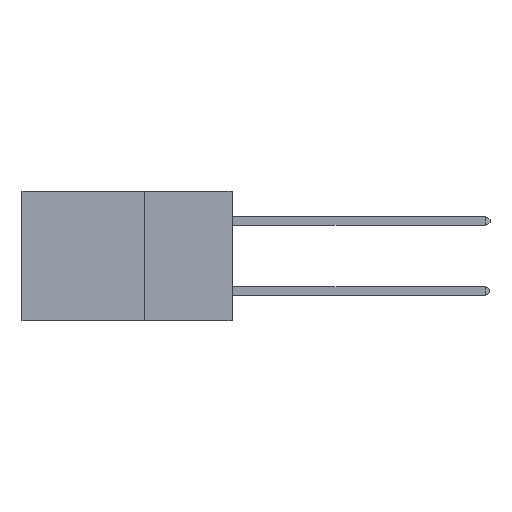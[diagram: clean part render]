
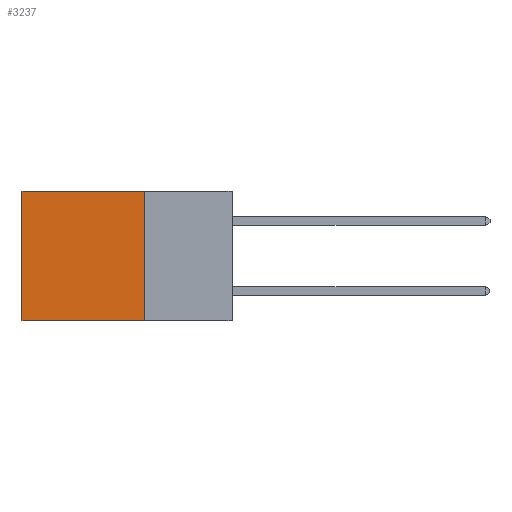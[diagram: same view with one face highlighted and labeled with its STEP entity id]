
A CAD part, left-side view. The second image highlights one B-rep face of the part: STEP entity #3237.
In plain terms, the highlighted planar face has unit normal (-1, 0, 0).
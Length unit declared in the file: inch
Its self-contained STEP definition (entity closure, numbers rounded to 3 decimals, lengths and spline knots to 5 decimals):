
#46 = VERTEX_POINT ( 'NONE', #4002 ) ;
#848 = DIRECTION ( 'NONE',  ( 1., 0., 0. ) ) ;
#983 = VECTOR ( 'NONE', #1542, 39.37008 ) ;
#1263 = VERTEX_POINT ( 'NONE', #14115 ) ;
#1542 = DIRECTION ( 'NONE',  ( 0., 0., -1. ) ) ;
#1640 = EDGE_LOOP ( 'NONE', ( #15507, #9626, #14512, #6989 ) ) ;
#1706 = EDGE_CURVE ( 'NONE', #14090, #1263, #13943, .T. ) ;
#1722 = VECTOR ( 'NONE', #9098, 39.37008 ) ;
#2102 = LINE ( 'NONE', #12699, #1722 ) ;
#3237 = ADVANCED_FACE ( 'NONE', ( #11643 ), #10571, .F. ) ;
#3840 = EDGE_CURVE ( 'NONE', #46, #14090, #14632, .T. ) ;
#4002 = CARTESIAN_POINT ( 'NONE',  ( 0.2875, 0.25, 0. ) ) ;
#6776 = CARTESIAN_POINT ( 'NONE',  ( 0.2875, 0.6, 0. ) ) ;
#6989 = ORIENTED_EDGE ( 'NONE', *, *, #3840, .T. ) ;
#8209 = CARTESIAN_POINT ( 'NONE',  ( 0.2875, 0.25, 0. ) ) ;
#9098 = DIRECTION ( 'NONE',  ( 0., 1., 0. ) ) ;
#9395 = DIRECTION ( 'NONE',  ( 0., 0., -1. ) ) ;
#9626 = ORIENTED_EDGE ( 'NONE', *, *, #9870, .F. ) ;
#9717 = AXIS2_PLACEMENT_3D ( 'NONE', #11804, #848, #9395 ) ;
#9870 = EDGE_CURVE ( 'NONE', #13954, #1263, #2102, .T. ) ;
#10298 = LINE ( 'NONE', #11307, #13118 ) ;
#10463 = EDGE_CURVE ( 'NONE', #46, #13954, #10298, .T. ) ;
#10571 = PLANE ( 'NONE',  #9717 ) ;
#11040 = VECTOR ( 'NONE', #15465, 39.37008 ) ;
#11307 = CARTESIAN_POINT ( 'NONE',  ( 0.2875, 0.25, 0. ) ) ;
#11643 = FACE_OUTER_BOUND ( 'NONE', #1640, .T. ) ;
#11804 = CARTESIAN_POINT ( 'NONE',  ( 0.2875, 0.25, 0. ) ) ;
#12522 = DIRECTION ( 'NONE',  ( 0., 0., -1. ) ) ;
#12699 = CARTESIAN_POINT ( 'NONE',  ( 0.2875, 0.25, -0.37 ) ) ;
#13118 = VECTOR ( 'NONE', #12522, 39.37008 ) ;
#13654 = CARTESIAN_POINT ( 'NONE',  ( 0.2875, 0.6, 0. ) ) ;
#13943 = LINE ( 'NONE', #13654, #983 ) ;
#13954 = VERTEX_POINT ( 'NONE', #15057 ) ;
#14090 = VERTEX_POINT ( 'NONE', #6776 ) ;
#14115 = CARTESIAN_POINT ( 'NONE',  ( 0.2875, 0.6, -0.37 ) ) ;
#14512 = ORIENTED_EDGE ( 'NONE', *, *, #10463, .F. ) ;
#14632 = LINE ( 'NONE', #8209, #11040 ) ;
#15057 = CARTESIAN_POINT ( 'NONE',  ( 0.2875, 0.25, -0.37 ) ) ;
#15465 = DIRECTION ( 'NONE',  ( 0., 1., 0. ) ) ;
#15507 = ORIENTED_EDGE ( 'NONE', *, *, #1706, .T. ) ;
